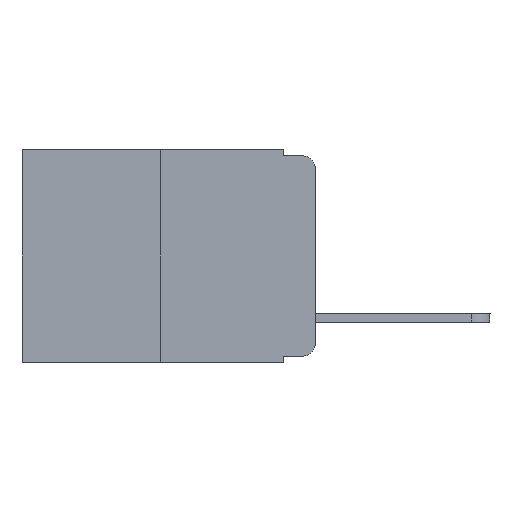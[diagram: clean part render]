
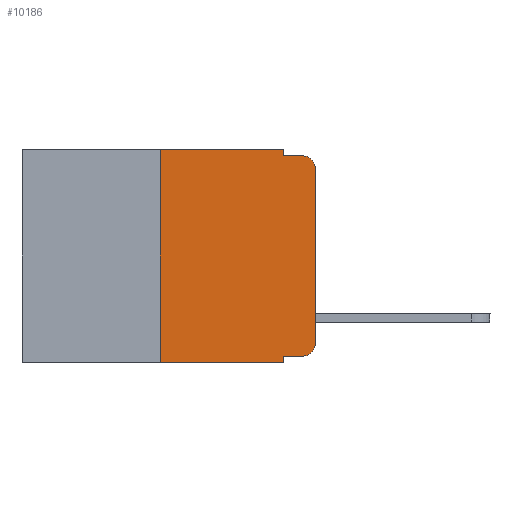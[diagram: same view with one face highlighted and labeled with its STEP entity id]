
A CAD part, left-side view. The second image highlights one B-rep face of the part: STEP entity #10186.
In plain terms, the highlighted planar face has unit normal (-1, 0, 0).
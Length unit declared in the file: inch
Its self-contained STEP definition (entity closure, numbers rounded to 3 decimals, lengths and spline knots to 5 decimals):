
#76 = LINE ( 'NONE', #1891, #4062 ) ;
#199 = LINE ( 'NONE', #5785, #7853 ) ;
#210 = EDGE_CURVE ( 'NONE', #1064, #5599, #9457, .T. ) ;
#380 = VECTOR ( 'NONE', #3977, 39.37008 ) ;
#382 = DIRECTION ( 'NONE',  ( 1., 0., 0. ) ) ;
#538 = ORIENTED_EDGE ( 'NONE', *, *, #5263, .F. ) ;
#617 = CARTESIAN_POINT ( 'NONE',  ( 0., 0.25, 0. ) ) ;
#655 = EDGE_CURVE ( 'NONE', #4265, #4074, #199, .T. ) ;
#663 = DIRECTION ( 'NONE',  ( 0., 0., 1. ) ) ;
#830 = LINE ( 'NONE', #7374, #7086 ) ;
#841 = AXIS2_PLACEMENT_3D ( 'NONE', #2630, #1844, #8220 ) ;
#1024 = CARTESIAN_POINT ( 'NONE',  ( 0., 0.051, -0.343 ) ) ;
#1064 = VERTEX_POINT ( 'NONE', #7264 ) ;
#1383 = CARTESIAN_POINT ( 'NONE',  ( 0., 0.051, 0. ) ) ;
#1637 = ORIENTED_EDGE ( 'NONE', *, *, #8370, .T. ) ;
#1661 = LINE ( 'NONE', #2546, #380 ) ;
#1725 = VERTEX_POINT ( 'NONE', #8773 ) ;
#1786 = EDGE_CURVE ( 'NONE', #2491, #1725, #1978, .T. ) ;
#1844 = DIRECTION ( 'NONE',  ( -1., 0., 0. ) ) ;
#1891 = CARTESIAN_POINT ( 'NONE',  ( 0., 0.473, 0. ) ) ;
#1978 = LINE ( 'NONE', #6779, #4889 ) ;
#2042 = LINE ( 'NONE', #9915, #4730 ) ;
#2302 = CARTESIAN_POINT ( 'NONE',  ( 0., 0.473, -0.343 ) ) ;
#2323 = VERTEX_POINT ( 'NONE', #7754 ) ;
#2491 = VERTEX_POINT ( 'NONE', #3108 ) ;
#2546 = CARTESIAN_POINT ( 'NONE',  ( 0., 0., 0. ) ) ;
#2630 = CARTESIAN_POINT ( 'NONE',  ( 0., 0.02, -0.313 ) ) ;
#3108 = CARTESIAN_POINT ( 'NONE',  ( 0., 0.051, -0.333 ) ) ;
#3190 = VERTEX_POINT ( 'NONE', #7438 ) ;
#3199 = CARTESIAN_POINT ( 'NONE',  ( 0., 0., -0.313 ) ) ;
#3205 = VECTOR ( 'NONE', #663, 39.37008 ) ;
#3325 = EDGE_CURVE ( 'NONE', #1725, #3711, #4187, .T. ) ;
#3380 = DIRECTION ( 'NONE',  ( 0., 0., -1. ) ) ;
#3518 = FACE_OUTER_BOUND ( 'NONE', #9954, .T. ) ;
#3537 = ORIENTED_EDGE ( 'NONE', *, *, #655, .F. ) ;
#3711 = VERTEX_POINT ( 'NONE', #3199 ) ;
#3977 = DIRECTION ( 'NONE',  ( 0., 0., 1. ) ) ;
#4062 = VECTOR ( 'NONE', #5087, 39.37008 ) ;
#4074 = VERTEX_POINT ( 'NONE', #8088 ) ;
#4187 = CIRCLE ( 'NONE', #841, 0.02 ) ;
#4265 = VERTEX_POINT ( 'NONE', #1383 ) ;
#4377 = CIRCLE ( 'NONE', #5054, 0.02 ) ;
#4730 = VECTOR ( 'NONE', #9237, 39.37008 ) ;
#4889 = VECTOR ( 'NONE', #7456, 39.37008 ) ;
#5001 = DIRECTION ( 'NONE',  ( 0., 0., -1. ) ) ;
#5054 = AXIS2_PLACEMENT_3D ( 'NONE', #7397, #9828, #5001 ) ;
#5087 = DIRECTION ( 'NONE',  ( 0., -1., 0. ) ) ;
#5200 = CARTESIAN_POINT ( 'NONE',  ( 0., 0.02, -0.01 ) ) ;
#5222 = ORIENTED_EDGE ( 'NONE', *, *, #5926, .T. ) ;
#5263 = EDGE_CURVE ( 'NONE', #1064, #3190, #7732, .T. ) ;
#5599 = VERTEX_POINT ( 'NONE', #1024 ) ;
#5760 = AXIS2_PLACEMENT_3D ( 'NONE', #7402, #382, #6651 ) ;
#5785 = CARTESIAN_POINT ( 'NONE',  ( 0., 0.051, 0. ) ) ;
#5926 = EDGE_CURVE ( 'NONE', #2323, #10227, #4377, .T. ) ;
#5976 = PLANE ( 'NONE',  #5760 ) ;
#6075 = DIRECTION ( 'NONE',  ( 0., -1., 0. ) ) ;
#6216 = EDGE_CURVE ( 'NONE', #3190, #4265, #76, .T. ) ;
#6651 = DIRECTION ( 'NONE',  ( 0., 0., -1. ) ) ;
#6779 = CARTESIAN_POINT ( 'NONE',  ( 0., 0.051, -0.333 ) ) ;
#6795 = ORIENTED_EDGE ( 'NONE', *, *, #9236, .F. ) ;
#7086 = VECTOR ( 'NONE', #8059, 39.37008 ) ;
#7264 = CARTESIAN_POINT ( 'NONE',  ( 0., 0.25, -0.343 ) ) ;
#7268 = ORIENTED_EDGE ( 'NONE', *, *, #3325, .T. ) ;
#7374 = CARTESIAN_POINT ( 'NONE',  ( 0., 0.051, -0.01 ) ) ;
#7397 = CARTESIAN_POINT ( 'NONE',  ( 0., 0.02, -0.03 ) ) ;
#7402 = CARTESIAN_POINT ( 'NONE',  ( 0., 0.473, 0. ) ) ;
#7438 = CARTESIAN_POINT ( 'NONE',  ( 0., 0.25, 0. ) ) ;
#7456 = DIRECTION ( 'NONE',  ( 0., -1., 0. ) ) ;
#7732 = LINE ( 'NONE', #617, #3205 ) ;
#7754 = CARTESIAN_POINT ( 'NONE',  ( 0., 0., -0.03 ) ) ;
#7853 = VECTOR ( 'NONE', #3380, 39.37008 ) ;
#7990 = VECTOR ( 'NONE', #6075, 39.37008 ) ;
#8059 = DIRECTION ( 'NONE',  ( 0., -1., 0. ) ) ;
#8062 = EDGE_CURVE ( 'NONE', #2491, #5599, #2042, .T. ) ;
#8088 = CARTESIAN_POINT ( 'NONE',  ( 0., 0.051, -0.01 ) ) ;
#8220 = DIRECTION ( 'NONE',  ( 0., 0., -1. ) ) ;
#8370 = EDGE_CURVE ( 'NONE', #3711, #2323, #1661, .T. ) ;
#8773 = CARTESIAN_POINT ( 'NONE',  ( 0., 0.02, -0.333 ) ) ;
#8881 = ORIENTED_EDGE ( 'NONE', *, *, #6216, .F. ) ;
#9026 = ORIENTED_EDGE ( 'NONE', *, *, #210, .T. ) ;
#9169 = ORIENTED_EDGE ( 'NONE', *, *, #1786, .T. ) ;
#9236 = EDGE_CURVE ( 'NONE', #4074, #10227, #830, .T. ) ;
#9237 = DIRECTION ( 'NONE',  ( 0., 0., -1. ) ) ;
#9457 = LINE ( 'NONE', #2302, #7990 ) ;
#9689 = ORIENTED_EDGE ( 'NONE', *, *, #8062, .F. ) ;
#9828 = DIRECTION ( 'NONE',  ( -1., 0., 0. ) ) ;
#9915 = CARTESIAN_POINT ( 'NONE',  ( 0., 0.051, 0. ) ) ;
#9954 = EDGE_LOOP ( 'NONE', ( #1637, #5222, #6795, #3537, #8881, #538, #9026, #9689, #9169, #7268 ) ) ;
#10186 = ADVANCED_FACE ( 'NONE', ( #3518 ), #5976, .F. ) ;
#10227 = VERTEX_POINT ( 'NONE', #5200 ) ;
